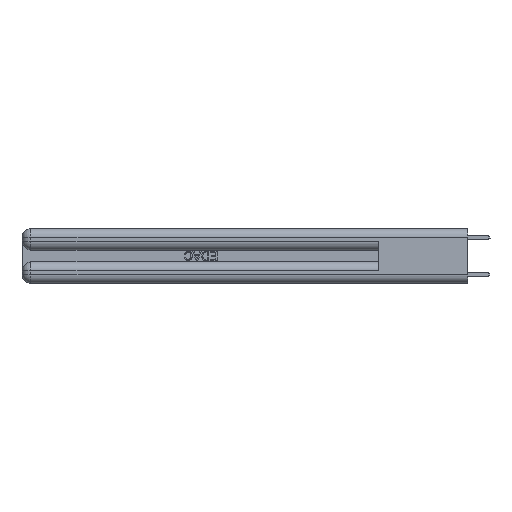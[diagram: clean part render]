
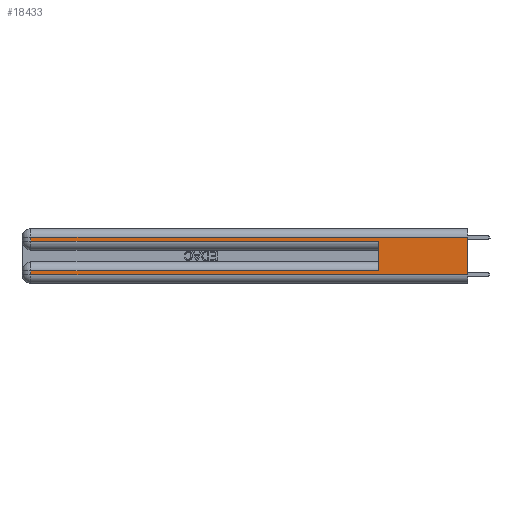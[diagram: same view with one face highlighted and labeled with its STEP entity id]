
A CAD part, left-side view. The second image highlights one B-rep face of the part: STEP entity #18433.
In plain terms, the highlighted planar face has unit normal (-1, 0, 0).
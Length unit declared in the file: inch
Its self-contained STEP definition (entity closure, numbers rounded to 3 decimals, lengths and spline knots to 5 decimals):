
#314 = VECTOR ( 'NONE', #15808, 39.37008 ) ;
#2244 = CARTESIAN_POINT ( 'NONE',  ( 0., 2.94, 0.085 ) ) ;
#2511 = CARTESIAN_POINT ( 'NONE',  ( 0., 0., 0.085 ) ) ;
#3618 = CARTESIAN_POINT ( 'NONE',  ( 0., 0., 0.37 ) ) ;
#4249 = VECTOR ( 'NONE', #20070, 39.37008 ) ;
#4634 = CARTESIAN_POINT ( 'NONE',  ( 0., 2.94, 0.285 ) ) ;
#4852 = ORIENTED_EDGE ( 'NONE', *, *, #23321, .T. ) ;
#4933 = CARTESIAN_POINT ( 'NONE',  ( 0., 0., 0.06 ) ) ;
#5206 = ORIENTED_EDGE ( 'NONE', *, *, #24278, .T. ) ;
#6204 = EDGE_CURVE ( 'NONE', #9188, #24812, #11691, .T. ) ;
#6217 = CARTESIAN_POINT ( 'NONE',  ( 0., 0., 0.06 ) ) ;
#6501 = CARTESIAN_POINT ( 'NONE',  ( 0., 0.6, 0.145 ) ) ;
#6972 = LINE ( 'NONE', #14271, #9222 ) ;
#7193 = EDGE_CURVE ( 'NONE', #29957, #24634, #20293, .T. ) ;
#7994 = ORIENTED_EDGE ( 'NONE', *, *, #15880, .T. ) ;
#8228 = EDGE_CURVE ( 'NONE', #11340, #9188, #6972, .T. ) ;
#8686 = DIRECTION ( 'NONE',  ( 0., 0., -1. ) ) ;
#8716 = LINE ( 'NONE', #10636, #4249 ) ;
#9188 = VERTEX_POINT ( 'NONE', #26155 ) ;
#9222 = VECTOR ( 'NONE', #8686, 39.37008 ) ;
#9843 = LINE ( 'NONE', #3618, #17216 ) ;
#10636 = CARTESIAN_POINT ( 'NONE',  ( 0., 2.94, 0.37 ) ) ;
#10684 = DIRECTION ( 'NONE',  ( 1., 0., 0. ) ) ;
#10714 = VERTEX_POINT ( 'NONE', #25939 ) ;
#10885 = DIRECTION ( 'NONE',  ( 0., 0., -1. ) ) ;
#11340 = VERTEX_POINT ( 'NONE', #2244 ) ;
#11691 = LINE ( 'NONE', #6217, #23456 ) ;
#12157 = EDGE_CURVE ( 'NONE', #29957, #11340, #22944, .T. ) ;
#12671 = DIRECTION ( 'NONE',  ( 0., 1., 0. ) ) ;
#13136 = ORIENTED_EDGE ( 'NONE', *, *, #8228, .T. ) ;
#14271 = CARTESIAN_POINT ( 'NONE',  ( 0., 2.94, 0.37 ) ) ;
#14874 = FACE_OUTER_BOUND ( 'NONE', #24861, .T. ) ;
#15808 = DIRECTION ( 'NONE',  ( 0., 0., 1. ) ) ;
#15880 = EDGE_CURVE ( 'NONE', #10714, #26785, #8716, .T. ) ;
#15906 = CARTESIAN_POINT ( 'NONE',  ( 0., 0.6, 0.285 ) ) ;
#16205 = LINE ( 'NONE', #27147, #28299 ) ;
#16361 = ORIENTED_EDGE ( 'NONE', *, *, #7193, .F. ) ;
#16434 = EDGE_CURVE ( 'NONE', #21576, #24812, #9843, .T. ) ;
#16868 = DIRECTION ( 'NONE',  ( 0., -1., 0. ) ) ;
#17216 = VECTOR ( 'NONE', #10885, 39.37008 ) ;
#17263 = ORIENTED_EDGE ( 'NONE', *, *, #6204, .T. ) ;
#17959 = VECTOR ( 'NONE', #16868, 39.37008 ) ;
#18404 = DIRECTION ( 'NONE',  ( 0., -1., 0. ) ) ;
#18433 = ADVANCED_FACE ( 'NONE', ( #14874 ), #24640, .F. ) ;
#19809 = ORIENTED_EDGE ( 'NONE', *, *, #12157, .T. ) ;
#20024 = DIRECTION ( 'NONE',  ( 0., 0., -1. ) ) ;
#20070 = DIRECTION ( 'NONE',  ( 0., 0., -1. ) ) ;
#20293 = LINE ( 'NONE', #6501, #314 ) ;
#21143 = ORIENTED_EDGE ( 'NONE', *, *, #16434, .F. ) ;
#21576 = VERTEX_POINT ( 'NONE', #26605 ) ;
#21716 = DIRECTION ( 'NONE',  ( 0., 1., 0. ) ) ;
#21874 = VECTOR ( 'NONE', #21716, 39.37008 ) ;
#22944 = LINE ( 'NONE', #2511, #21874 ) ;
#23321 = EDGE_CURVE ( 'NONE', #21576, #10714, #16205, .T. ) ;
#23456 = VECTOR ( 'NONE', #18404, 39.37008 ) ;
#23612 = CARTESIAN_POINT ( 'NONE',  ( 0., 0., 0.285 ) ) ;
#24173 = AXIS2_PLACEMENT_3D ( 'NONE', #24545, #10684, #20024 ) ;
#24278 = EDGE_CURVE ( 'NONE', #26785, #24634, #25659, .T. ) ;
#24545 = CARTESIAN_POINT ( 'NONE',  ( 0., 0., 0.37 ) ) ;
#24634 = VERTEX_POINT ( 'NONE', #15906 ) ;
#24640 = PLANE ( 'NONE',  #24173 ) ;
#24812 = VERTEX_POINT ( 'NONE', #4933 ) ;
#24861 = EDGE_LOOP ( 'NONE', ( #21143, #4852, #7994, #5206, #16361, #19809, #13136, #17263 ) ) ;
#25659 = LINE ( 'NONE', #23612, #17959 ) ;
#25939 = CARTESIAN_POINT ( 'NONE',  ( 0., 2.94, 0.31 ) ) ;
#26155 = CARTESIAN_POINT ( 'NONE',  ( 0., 2.94, 0.06 ) ) ;
#26605 = CARTESIAN_POINT ( 'NONE',  ( 0., 0., 0.31 ) ) ;
#26785 = VERTEX_POINT ( 'NONE', #4634 ) ;
#27147 = CARTESIAN_POINT ( 'NONE',  ( 0., 0., 0.31 ) ) ;
#28299 = VECTOR ( 'NONE', #12671, 39.37008 ) ;
#28751 = CARTESIAN_POINT ( 'NONE',  ( 0., 0.6, 0.085 ) ) ;
#29957 = VERTEX_POINT ( 'NONE', #28751 ) ;
